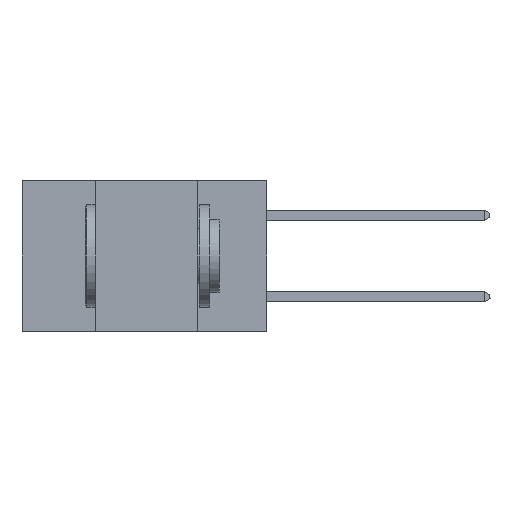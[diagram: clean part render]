
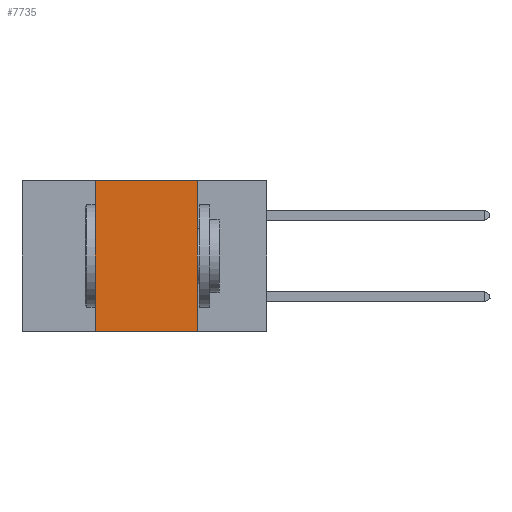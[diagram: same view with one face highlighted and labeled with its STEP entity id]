
A CAD part, left-side view. The second image highlights one B-rep face of the part: STEP entity #7735.
In plain terms, the highlighted planar face has unit normal (-1, 0, 0).
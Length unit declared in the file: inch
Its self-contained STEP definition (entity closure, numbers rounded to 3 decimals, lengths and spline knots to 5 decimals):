
#1340 = ORIENTED_EDGE ( 'NONE', *, *, #10826, .F. ) ;
#2421 = FACE_OUTER_BOUND ( 'NONE', #34169, .T. ) ;
#2953 = VERTEX_POINT ( 'NONE', #4726 ) ;
#3190 = VERTEX_POINT ( 'NONE', #16354 ) ;
#3299 = PLANE ( 'NONE',  #11246 ) ;
#4281 = LINE ( 'NONE', #4718, #31227 ) ;
#4718 = CARTESIAN_POINT ( 'NONE',  ( 0., 0.17, 0. ) ) ;
#4726 = CARTESIAN_POINT ( 'NONE',  ( 0., 0.42, 0. ) ) ;
#7042 = DIRECTION ( 'NONE',  ( 1., 0., 0. ) ) ;
#7731 = EDGE_CURVE ( 'NONE', #31083, #3190, #23066, .T. ) ;
#7735 = ADVANCED_FACE ( 'NONE', ( #2421 ), #3299, .F. ) ;
#10204 = EDGE_CURVE ( 'NONE', #36535, #3190, #4281, .T. ) ;
#10367 = DIRECTION ( 'NONE',  ( 0., -1., 0. ) ) ;
#10826 = EDGE_CURVE ( 'NONE', #31083, #2953, #42610, .T. ) ;
#11083 = CARTESIAN_POINT ( 'NONE',  ( 0., 0.17, 0. ) ) ;
#11246 = AXIS2_PLACEMENT_3D ( 'NONE', #17059, #7042, #20102 ) ;
#14565 = DIRECTION ( 'NONE',  ( 0., 0., -1. ) ) ;
#14899 = LINE ( 'NONE', #19048, #40784 ) ;
#16354 = CARTESIAN_POINT ( 'NONE',  ( 0., 0.17, -0.37 ) ) ;
#17059 = CARTESIAN_POINT ( 'NONE',  ( 0., 0.6, 0. ) ) ;
#19048 = CARTESIAN_POINT ( 'NONE',  ( 0., 0.6, 0. ) ) ;
#20102 = DIRECTION ( 'NONE',  ( 0., 0., -1. ) ) ;
#22100 = VECTOR ( 'NONE', #10367, 39.37008 ) ;
#23066 = LINE ( 'NONE', #33275, #22100 ) ;
#25533 = DIRECTION ( 'NONE',  ( 0., -1., 0. ) ) ;
#26499 = CARTESIAN_POINT ( 'NONE',  ( 0., 0.42, -0.37 ) ) ;
#26653 = ORIENTED_EDGE ( 'NONE', *, *, #32874, .F. ) ;
#30260 = ORIENTED_EDGE ( 'NONE', *, *, #7731, .T. ) ;
#30668 = ORIENTED_EDGE ( 'NONE', *, *, #10204, .F. ) ;
#30889 = DIRECTION ( 'NONE',  ( 0., 0., 1. ) ) ;
#31083 = VERTEX_POINT ( 'NONE', #26499 ) ;
#31227 = VECTOR ( 'NONE', #14565, 39.37008 ) ;
#32874 = EDGE_CURVE ( 'NONE', #2953, #36535, #14899, .T. ) ;
#33275 = CARTESIAN_POINT ( 'NONE',  ( 0., 0.6, -0.37 ) ) ;
#34169 = EDGE_LOOP ( 'NONE', ( #30668, #26653, #1340, #30260 ) ) ;
#36535 = VERTEX_POINT ( 'NONE', #11083 ) ;
#37380 = CARTESIAN_POINT ( 'NONE',  ( 0., 0.42, 0. ) ) ;
#40784 = VECTOR ( 'NONE', #25533, 39.37008 ) ;
#41563 = VECTOR ( 'NONE', #30889, 39.37008 ) ;
#42610 = LINE ( 'NONE', #37380, #41563 ) ;
